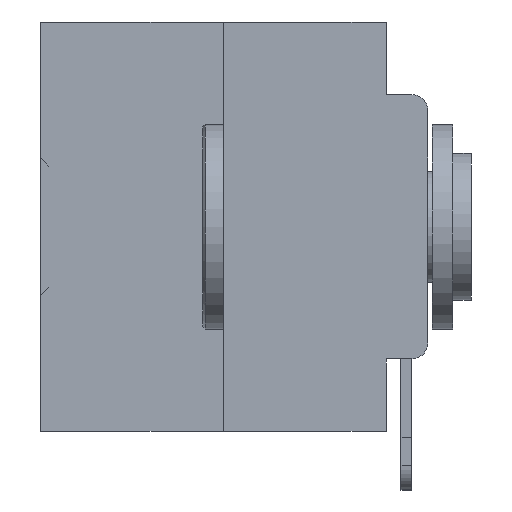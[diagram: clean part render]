
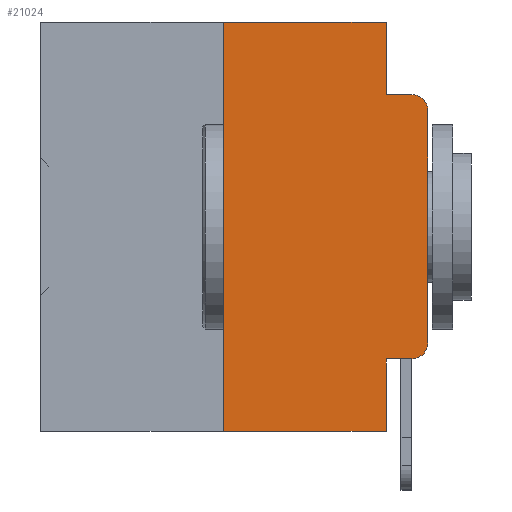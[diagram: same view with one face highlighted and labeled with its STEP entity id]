
A CAD part, left-side view. The second image highlights one B-rep face of the part: STEP entity #21024.
In plain terms, the highlighted planar face has unit normal (-1, 0, 0).
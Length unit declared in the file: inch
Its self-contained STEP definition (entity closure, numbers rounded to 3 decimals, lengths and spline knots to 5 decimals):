
#270 = CARTESIAN_POINT ( 'NONE',  ( 0., 0.051, -0.5 ) ) ;
#388 = DIRECTION ( 'NONE',  ( 0., 0., -1. ) ) ;
#535 = VECTOR ( 'NONE', #34707, 39.37008 ) ;
#1010 = VECTOR ( 'NONE', #8965, 39.37008 ) ;
#1146 = VERTEX_POINT ( 'NONE', #270 ) ;
#1198 = ORIENTED_EDGE ( 'NONE', *, *, #17317, .T. ) ;
#1648 = VECTOR ( 'NONE', #37259, 39.37008 ) ;
#1792 = VERTEX_POINT ( 'NONE', #12449 ) ;
#1884 = CARTESIAN_POINT ( 'NONE',  ( 0., 0.051, -0.0885 ) ) ;
#2337 = DIRECTION ( 'NONE',  ( 0., -1., 0. ) ) ;
#2743 = DIRECTION ( 'NONE',  ( 0., 0., 1. ) ) ;
#2989 = CARTESIAN_POINT ( 'NONE',  ( 0., 0.051, -0.4115 ) ) ;
#3848 = CARTESIAN_POINT ( 'NONE',  ( 0., 0., -0.1085 ) ) ;
#4653 = VECTOR ( 'NONE', #14560, 39.37008 ) ;
#5523 = DIRECTION ( 'NONE',  ( -1., 0., 0. ) ) ;
#5545 = VERTEX_POINT ( 'NONE', #1884 ) ;
#6166 = DIRECTION ( 'NONE',  ( 0., -1., 0. ) ) ;
#6253 = LINE ( 'NONE', #20860, #21475 ) ;
#7600 = CARTESIAN_POINT ( 'NONE',  ( 0., 0.051, 0. ) ) ;
#7903 = CARTESIAN_POINT ( 'NONE',  ( 0., 0.25, 0. ) ) ;
#8234 = VERTEX_POINT ( 'NONE', #13568 ) ;
#8261 = LINE ( 'NONE', #32713, #38402 ) ;
#8430 = EDGE_CURVE ( 'NONE', #29083, #9616, #20329, .T. ) ;
#8871 = LINE ( 'NONE', #7600, #535 ) ;
#8952 = AXIS2_PLACEMENT_3D ( 'NONE', #17349, #38347, #20404 ) ;
#8965 = DIRECTION ( 'NONE',  ( 0., 0., 1. ) ) ;
#9616 = VERTEX_POINT ( 'NONE', #34803 ) ;
#9971 = ORIENTED_EDGE ( 'NONE', *, *, #31392, .F. ) ;
#10277 = LINE ( 'NONE', #27000, #1010 ) ;
#10494 = EDGE_CURVE ( 'NONE', #24451, #29083, #10277, .T. ) ;
#12325 = ORIENTED_EDGE ( 'NONE', *, *, #10494, .T. ) ;
#12449 = CARTESIAN_POINT ( 'NONE',  ( 0., 0.25, -0.5 ) ) ;
#12970 = CARTESIAN_POINT ( 'NONE',  ( 0., 0., -0.3915 ) ) ;
#13092 = CARTESIAN_POINT ( 'NONE',  ( 0., 0.473, -0.5 ) ) ;
#13478 = CIRCLE ( 'NONE', #8952, 0.02 ) ;
#13568 = CARTESIAN_POINT ( 'NONE',  ( 0., 0.02, -0.4115 ) ) ;
#13600 = AXIS2_PLACEMENT_3D ( 'NONE', #23689, #5523, #26670 ) ;
#14223 = ORIENTED_EDGE ( 'NONE', *, *, #37448, .F. ) ;
#14560 = DIRECTION ( 'NONE',  ( 0., 0., -1. ) ) ;
#15302 = EDGE_CURVE ( 'NONE', #8234, #24451, #13478, .T. ) ;
#15307 = CARTESIAN_POINT ( 'NONE',  ( 0., 0.051, 0. ) ) ;
#15642 = PLANE ( 'NONE',  #18994 ) ;
#17317 = EDGE_CURVE ( 'NONE', #18272, #8234, #38201, .T. ) ;
#17349 = CARTESIAN_POINT ( 'NONE',  ( 0., 0.02, -0.3915 ) ) ;
#18033 = ORIENTED_EDGE ( 'NONE', *, *, #30401, .T. ) ;
#18272 = VERTEX_POINT ( 'NONE', #18927 ) ;
#18831 = DIRECTION ( 'NONE',  ( 1., 0., 0. ) ) ;
#18927 = CARTESIAN_POINT ( 'NONE',  ( 0., 0.051, -0.4115 ) ) ;
#18949 = LINE ( 'NONE', #13092, #1648 ) ;
#18994 = AXIS2_PLACEMENT_3D ( 'NONE', #33735, #18831, #388 ) ;
#19035 = FACE_OUTER_BOUND ( 'NONE', #25100, .T. ) ;
#20329 = CIRCLE ( 'NONE', #13600, 0.02 ) ;
#20404 = DIRECTION ( 'NONE',  ( 0., 0., -1. ) ) ;
#20860 = CARTESIAN_POINT ( 'NONE',  ( 0., 0.051, -0.0885 ) ) ;
#20876 = LINE ( 'NONE', #32540, #4653 ) ;
#21024 = ADVANCED_FACE ( 'NONE', ( #19035 ), #15642, .F. ) ;
#21387 = EDGE_CURVE ( 'NONE', #18272, #1146, #20876, .T. ) ;
#21475 = VECTOR ( 'NONE', #32879, 39.37008 ) ;
#23607 = VECTOR ( 'NONE', #2743, 39.37008 ) ;
#23689 = CARTESIAN_POINT ( 'NONE',  ( 0., 0.02, -0.1085 ) ) ;
#24451 = VERTEX_POINT ( 'NONE', #12970 ) ;
#25100 = EDGE_LOOP ( 'NONE', ( #12325, #36302, #14223, #38188, #39124, #9971, #18033, #29719, #1198, #33497 ) ) ;
#26670 = DIRECTION ( 'NONE',  ( 0., 0., -1. ) ) ;
#27000 = CARTESIAN_POINT ( 'NONE',  ( 0., 0., 0. ) ) ;
#27412 = EDGE_CURVE ( 'NONE', #34859, #28242, #8261, .T. ) ;
#28242 = VERTEX_POINT ( 'NONE', #15307 ) ;
#29083 = VERTEX_POINT ( 'NONE', #3848 ) ;
#29719 = ORIENTED_EDGE ( 'NONE', *, *, #21387, .F. ) ;
#29933 = CARTESIAN_POINT ( 'NONE',  ( 0., 0.25, 0. ) ) ;
#30200 = VECTOR ( 'NONE', #6166, 39.37008 ) ;
#30401 = EDGE_CURVE ( 'NONE', #1792, #1146, #18949, .T. ) ;
#30617 = LINE ( 'NONE', #29933, #23607 ) ;
#31392 = EDGE_CURVE ( 'NONE', #1792, #34859, #30617, .T. ) ;
#32540 = CARTESIAN_POINT ( 'NONE',  ( 0., 0.051, 0. ) ) ;
#32713 = CARTESIAN_POINT ( 'NONE',  ( 0., 0.473, 0. ) ) ;
#32879 = DIRECTION ( 'NONE',  ( 0., -1., 0. ) ) ;
#33497 = ORIENTED_EDGE ( 'NONE', *, *, #15302, .T. ) ;
#33735 = CARTESIAN_POINT ( 'NONE',  ( 0., 0.473, 0. ) ) ;
#34707 = DIRECTION ( 'NONE',  ( 0., 0., -1. ) ) ;
#34803 = CARTESIAN_POINT ( 'NONE',  ( 0., 0.02, -0.0885 ) ) ;
#34859 = VERTEX_POINT ( 'NONE', #7903 ) ;
#35420 = EDGE_CURVE ( 'NONE', #28242, #5545, #8871, .T. ) ;
#36302 = ORIENTED_EDGE ( 'NONE', *, *, #8430, .T. ) ;
#37259 = DIRECTION ( 'NONE',  ( 0., -1., 0. ) ) ;
#37448 = EDGE_CURVE ( 'NONE', #5545, #9616, #6253, .T. ) ;
#38188 = ORIENTED_EDGE ( 'NONE', *, *, #35420, .F. ) ;
#38201 = LINE ( 'NONE', #2989, #30200 ) ;
#38347 = DIRECTION ( 'NONE',  ( -1., 0., 0. ) ) ;
#38402 = VECTOR ( 'NONE', #2337, 39.37008 ) ;
#39124 = ORIENTED_EDGE ( 'NONE', *, *, #27412, .F. ) ;
